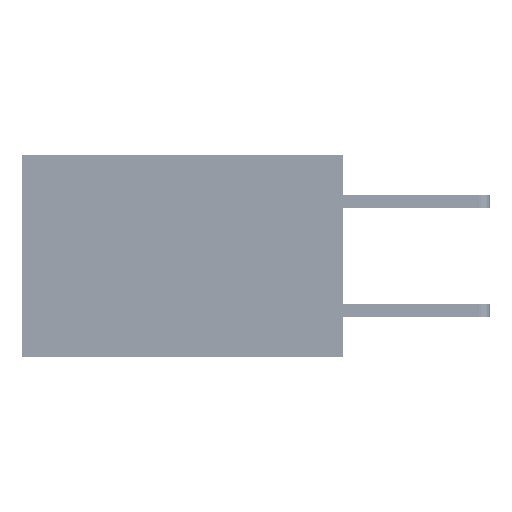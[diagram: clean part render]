
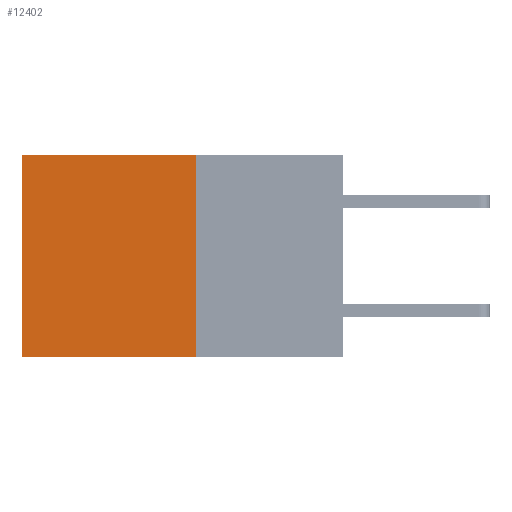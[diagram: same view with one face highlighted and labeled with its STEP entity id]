
A CAD part, left-side view. The second image highlights one B-rep face of the part: STEP entity #12402.
In plain terms, the highlighted planar face has unit normal (-1, 0, 0).
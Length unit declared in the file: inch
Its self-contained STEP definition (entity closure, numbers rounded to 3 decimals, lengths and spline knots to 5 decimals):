
#257 = VERTEX_POINT ( 'NONE', #16861 ) ;
#538 = VECTOR ( 'NONE', #16167, 39.37008 ) ;
#1068 = CARTESIAN_POINT ( 'NONE',  ( 0.277, 0.59, -0.37 ) ) ;
#2071 = LINE ( 'NONE', #26535, #538 ) ;
#2871 = VECTOR ( 'NONE', #5238, 39.37008 ) ;
#3611 = FACE_OUTER_BOUND ( 'NONE', #29672, .T. ) ;
#5238 = DIRECTION ( 'NONE',  ( 0., 0., -1. ) ) ;
#5360 = ORIENTED_EDGE ( 'NONE', *, *, #14091, .T. ) ;
#5789 = EDGE_CURVE ( 'NONE', #257, #10966, #2071, .T. ) ;
#8790 = LINE ( 'NONE', #19678, #34551 ) ;
#10949 = LINE ( 'NONE', #29686, #2871 ) ;
#10966 = VERTEX_POINT ( 'NONE', #1068 ) ;
#11646 = DIRECTION ( 'NONE',  ( 0., 1., 0. ) ) ;
#12402 = ADVANCED_FACE ( 'NONE', ( #3611 ), #25771, .F. ) ;
#13943 = VERTEX_POINT ( 'NONE', #20235 ) ;
#14091 = EDGE_CURVE ( 'NONE', #25289, #10966, #10949, .T. ) ;
#16167 = DIRECTION ( 'NONE',  ( 0., 1., 0. ) ) ;
#16861 = CARTESIAN_POINT ( 'NONE',  ( 0.277, 0.27, -0.37 ) ) ;
#17360 = CARTESIAN_POINT ( 'NONE',  ( 0.277, 0.27, -0.37 ) ) ;
#17631 = AXIS2_PLACEMENT_3D ( 'NONE', #17360, #20046, #31945 ) ;
#18963 = ORIENTED_EDGE ( 'NONE', *, *, #27717, .F. ) ;
#19344 = ORIENTED_EDGE ( 'NONE', *, *, #5789, .F. ) ;
#19678 = CARTESIAN_POINT ( 'NONE',  ( 0.277, 0.27, 0. ) ) ;
#20046 = DIRECTION ( 'NONE',  ( 1., 0., 0. ) ) ;
#20235 = CARTESIAN_POINT ( 'NONE',  ( 0.277, 0.27, 0. ) ) ;
#21660 = CARTESIAN_POINT ( 'NONE',  ( 0.277, 0.27, -0.37 ) ) ;
#23814 = LINE ( 'NONE', #21660, #31618 ) ;
#25289 = VERTEX_POINT ( 'NONE', #25866 ) ;
#25771 = PLANE ( 'NONE',  #17631 ) ;
#25822 = DIRECTION ( 'NONE',  ( 0., 0., -1. ) ) ;
#25866 = CARTESIAN_POINT ( 'NONE',  ( 0.277, 0.59, 0. ) ) ;
#26535 = CARTESIAN_POINT ( 'NONE',  ( 0.277, 0.27, -0.37 ) ) ;
#27717 = EDGE_CURVE ( 'NONE', #13943, #257, #23814, .T. ) ;
#28278 = ORIENTED_EDGE ( 'NONE', *, *, #29799, .T. ) ;
#29672 = EDGE_LOOP ( 'NONE', ( #5360, #19344, #18963, #28278 ) ) ;
#29686 = CARTESIAN_POINT ( 'NONE',  ( 0.277, 0.59, -0.37 ) ) ;
#29799 = EDGE_CURVE ( 'NONE', #13943, #25289, #8790, .T. ) ;
#31618 = VECTOR ( 'NONE', #25822, 39.37008 ) ;
#31945 = DIRECTION ( 'NONE',  ( 0., 0., -1. ) ) ;
#34551 = VECTOR ( 'NONE', #11646, 39.37008 ) ;
